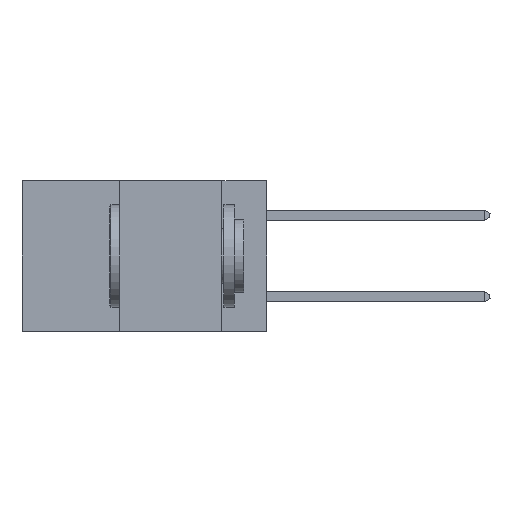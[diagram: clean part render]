
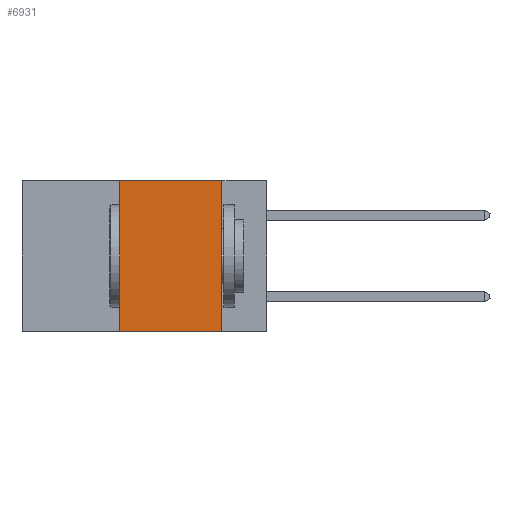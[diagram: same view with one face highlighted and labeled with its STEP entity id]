
A CAD part, left-side view. The second image highlights one B-rep face of the part: STEP entity #6931.
In plain terms, the highlighted planar face has unit normal (-1, 0, 0).
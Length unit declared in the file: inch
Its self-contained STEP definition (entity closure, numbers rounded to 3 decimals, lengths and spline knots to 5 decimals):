
#520 = DIRECTION ( 'NONE',  ( 0., 0., -1. ) ) ;
#908 = CARTESIAN_POINT ( 'NONE',  ( 0., 0.36, 0. ) ) ;
#1500 = EDGE_CURVE ( 'NONE', #14395, #19290, #16199, .T. ) ;
#2034 = VECTOR ( 'NONE', #5589, 39.37008 ) ;
#2740 = EDGE_CURVE ( 'NONE', #14395, #11082, #5937, .T. ) ;
#2901 = ORIENTED_EDGE ( 'NONE', *, *, #2740, .F. ) ;
#3335 = CARTESIAN_POINT ( 'NONE',  ( 0., 0.11, -0.37 ) ) ;
#3833 = VERTEX_POINT ( 'NONE', #17982 ) ;
#3901 = CARTESIAN_POINT ( 'NONE',  ( 0., 0.36, 0. ) ) ;
#4160 = DIRECTION ( 'NONE',  ( 0., 0., 1. ) ) ;
#4228 = LINE ( 'NONE', #13498, #21682 ) ;
#4402 = EDGE_LOOP ( 'NONE', ( #8770, #14520, #2901, #14602 ) ) ;
#5589 = DIRECTION ( 'NONE',  ( 0., -1., 0. ) ) ;
#5742 = CARTESIAN_POINT ( 'NONE',  ( 0., 0.6, -0.37 ) ) ;
#5937 = LINE ( 'NONE', #3901, #14787 ) ;
#6047 = CARTESIAN_POINT ( 'NONE',  ( 0., 0.6, 0. ) ) ;
#6348 = EDGE_CURVE ( 'NONE', #3833, #19290, #9942, .T. ) ;
#6931 = ADVANCED_FACE ( 'NONE', ( #21492 ), #16609, .F. ) ;
#8409 = CARTESIAN_POINT ( 'NONE',  ( 0., 0.36, -0.37 ) ) ;
#8473 = EDGE_CURVE ( 'NONE', #11082, #3833, #4228, .T. ) ;
#8770 = ORIENTED_EDGE ( 'NONE', *, *, #6348, .F. ) ;
#9669 = DIRECTION ( 'NONE',  ( 0., 0., -1. ) ) ;
#9942 = LINE ( 'NONE', #14802, #22555 ) ;
#11082 = VERTEX_POINT ( 'NONE', #908 ) ;
#11911 = AXIS2_PLACEMENT_3D ( 'NONE', #6047, #20035, #9669 ) ;
#13498 = CARTESIAN_POINT ( 'NONE',  ( 0., 0.6, 0. ) ) ;
#14395 = VERTEX_POINT ( 'NONE', #8409 ) ;
#14520 = ORIENTED_EDGE ( 'NONE', *, *, #8473, .F. ) ;
#14602 = ORIENTED_EDGE ( 'NONE', *, *, #1500, .T. ) ;
#14787 = VECTOR ( 'NONE', #4160, 39.37008 ) ;
#14802 = CARTESIAN_POINT ( 'NONE',  ( 0., 0.11, 0. ) ) ;
#15267 = DIRECTION ( 'NONE',  ( 0., -1., 0. ) ) ;
#16199 = LINE ( 'NONE', #5742, #2034 ) ;
#16609 = PLANE ( 'NONE',  #11911 ) ;
#17982 = CARTESIAN_POINT ( 'NONE',  ( 0., 0.11, 0. ) ) ;
#19290 = VERTEX_POINT ( 'NONE', #3335 ) ;
#20035 = DIRECTION ( 'NONE',  ( 1., 0., 0. ) ) ;
#21492 = FACE_OUTER_BOUND ( 'NONE', #4402, .T. ) ;
#21682 = VECTOR ( 'NONE', #15267, 39.37008 ) ;
#22555 = VECTOR ( 'NONE', #520, 39.37008 ) ;
